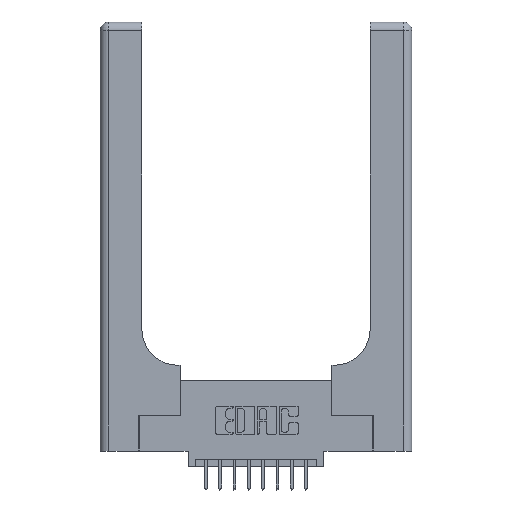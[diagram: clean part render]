
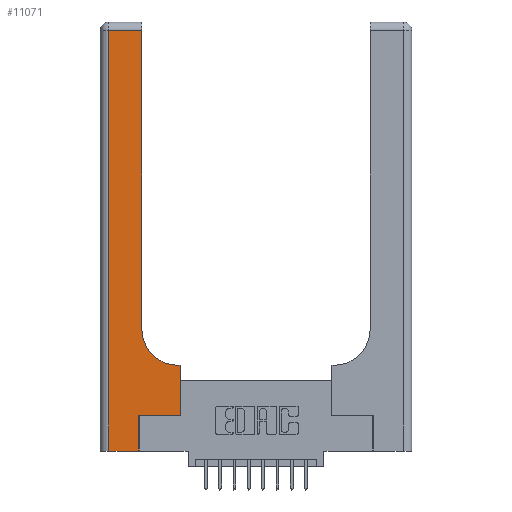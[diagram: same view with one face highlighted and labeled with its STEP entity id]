
A CAD part, top view. The second image highlights one B-rep face of the part: STEP entity #11071.
In plain terms, the highlighted planar face has unit normal (0, 0, 1).
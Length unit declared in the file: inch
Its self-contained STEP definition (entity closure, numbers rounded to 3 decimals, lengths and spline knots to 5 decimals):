
#88 = VERTEX_POINT ( 'NONE', #7089 ) ;
#295 = VECTOR ( 'NONE', #4574, 39.37008 ) ;
#316 = EDGE_CURVE ( 'NONE', #15069, #2921, #8820, .T. ) ;
#520 = PLANE ( 'NONE',  #4852 ) ;
#888 = LINE ( 'NONE', #1332, #7542 ) ;
#951 = EDGE_CURVE ( 'NONE', #16034, #15922, #11144, .T. ) ;
#986 = EDGE_CURVE ( 'NONE', #9569, #9562, #5456, .T. ) ;
#1092 = ORIENTED_EDGE ( 'NONE', *, *, #16101, .T. ) ;
#1332 = CARTESIAN_POINT ( 'NONE',  ( 0.2915, 3., 0.37 ) ) ;
#1518 = EDGE_CURVE ( 'NONE', #2921, #11020, #15280, .T. ) ;
#1629 = CARTESIAN_POINT ( 'NONE',  ( 0.06, 0., 0.37 ) ) ;
#1676 = DIRECTION ( 'NONE',  ( 0., 0., -1. ) ) ;
#2145 = DIRECTION ( 'NONE',  ( -1., 0., 0. ) ) ;
#2536 = VECTOR ( 'NONE', #2145, 39.37008 ) ;
#2921 = VERTEX_POINT ( 'NONE', #11684 ) ;
#4001 = CARTESIAN_POINT ( 'NONE',  ( 0.269, 0., 0.37 ) ) ;
#4333 = DIRECTION ( 'NONE',  ( -1., 0., 0. ) ) ;
#4574 = DIRECTION ( 'NONE',  ( 1., 0., 0. ) ) ;
#4661 = VECTOR ( 'NONE', #15684, 39.37008 ) ;
#4852 = AXIS2_PLACEMENT_3D ( 'NONE', #9300, #1676, #13098 ) ;
#4857 = VECTOR ( 'NONE', #5450, 39.37008 ) ;
#4906 = ORIENTED_EDGE ( 'NONE', *, *, #316, .T. ) ;
#5363 = DIRECTION ( 'NONE',  ( 1., 0., 0. ) ) ;
#5450 = DIRECTION ( 'NONE',  ( 0., -1., 0. ) ) ;
#5456 = LINE ( 'NONE', #9406, #4661 ) ;
#5468 = ORIENTED_EDGE ( 'NONE', *, *, #986, .T. ) ;
#5561 = VERTEX_POINT ( 'NONE', #4001 ) ;
#6009 = VECTOR ( 'NONE', #11252, 39.37008 ) ;
#6308 = DIRECTION ( 'NONE',  ( 0., 1., 0. ) ) ;
#6464 = CARTESIAN_POINT ( 'NONE',  ( 0.5585, 0.25, 0.37 ) ) ;
#6679 = CARTESIAN_POINT ( 'NONE',  ( 0., 2.94, 0.37 ) ) ;
#7070 = CARTESIAN_POINT ( 'NONE',  ( 0.2915, 0.6, 0.37 ) ) ;
#7089 = CARTESIAN_POINT ( 'NONE',  ( 0.2915, 2.94, 0.37 ) ) ;
#7542 = VECTOR ( 'NONE', #6308, 39.37008 ) ;
#7837 = CARTESIAN_POINT ( 'NONE',  ( 0.5415, 0.85, 0.37 ) ) ;
#7860 = LINE ( 'NONE', #6679, #16120 ) ;
#7873 = CARTESIAN_POINT ( 'NONE',  ( 0.06, 3., 0.37 ) ) ;
#7876 = VECTOR ( 'NONE', #11404, 39.37008 ) ;
#8270 = LINE ( 'NONE', #6464, #7876 ) ;
#8290 = EDGE_LOOP ( 'NONE', ( #9722, #14265, #12399, #10704, #1092, #5468, #15991, #4906, #9548 ) ) ;
#8411 = CARTESIAN_POINT ( 'NONE',  ( 0.269, 0., 0.37 ) ) ;
#8820 = LINE ( 'NONE', #7070, #2536 ) ;
#9149 = CARTESIAN_POINT ( 'NONE',  ( 0.269, 0.25, 0.37 ) ) ;
#9300 = CARTESIAN_POINT ( 'NONE',  ( 0., 3., 0.37 ) ) ;
#9326 = LINE ( 'NONE', #10823, #295 ) ;
#9406 = CARTESIAN_POINT ( 'NONE',  ( 0.269, 0.25, 0.37 ) ) ;
#9500 = CARTESIAN_POINT ( 'NONE',  ( 0.5585, 0.6, 0.37 ) ) ;
#9548 = ORIENTED_EDGE ( 'NONE', *, *, #1518, .T. ) ;
#9562 = VERTEX_POINT ( 'NONE', #10160 ) ;
#9569 = VERTEX_POINT ( 'NONE', #9149 ) ;
#9588 = EDGE_CURVE ( 'NONE', #15922, #5561, #9326, .T. ) ;
#9722 = ORIENTED_EDGE ( 'NONE', *, *, #16256, .T. ) ;
#10160 = CARTESIAN_POINT ( 'NONE',  ( 0.5585, 0.25, 0.37 ) ) ;
#10704 = ORIENTED_EDGE ( 'NONE', *, *, #9588, .T. ) ;
#10823 = CARTESIAN_POINT ( 'NONE',  ( 0., 0., 0.37 ) ) ;
#11020 = VERTEX_POINT ( 'NONE', #14228 ) ;
#11071 = ADVANCED_FACE ( 'NONE', ( #13222 ), #520, .F. ) ;
#11144 = LINE ( 'NONE', #7873, #4857 ) ;
#11252 = DIRECTION ( 'NONE',  ( 0., 1., 0. ) ) ;
#11404 = DIRECTION ( 'NONE',  ( 0., 1., 0. ) ) ;
#11684 = CARTESIAN_POINT ( 'NONE',  ( 0.5415, 0.6, 0.37 ) ) ;
#12010 = EDGE_CURVE ( 'NONE', #9562, #15069, #8270, .T. ) ;
#12242 = EDGE_CURVE ( 'NONE', #88, #16034, #7860, .T. ) ;
#12399 = ORIENTED_EDGE ( 'NONE', *, *, #951, .T. ) ;
#12736 = DIRECTION ( 'NONE',  ( 0., 0., -1. ) ) ;
#12802 = AXIS2_PLACEMENT_3D ( 'NONE', #7837, #12736, #5363 ) ;
#13098 = DIRECTION ( 'NONE',  ( -1., 0., 0. ) ) ;
#13222 = FACE_OUTER_BOUND ( 'NONE', #8290, .T. ) ;
#13919 = LINE ( 'NONE', #8411, #6009 ) ;
#14228 = CARTESIAN_POINT ( 'NONE',  ( 0.2915, 0.85, 0.37 ) ) ;
#14265 = ORIENTED_EDGE ( 'NONE', *, *, #12242, .T. ) ;
#15069 = VERTEX_POINT ( 'NONE', #9500 ) ;
#15280 = CIRCLE ( 'NONE', #12802, 0.25 ) ;
#15684 = DIRECTION ( 'NONE',  ( 1., 0., 0. ) ) ;
#15901 = CARTESIAN_POINT ( 'NONE',  ( 0.06, 2.94, 0.37 ) ) ;
#15922 = VERTEX_POINT ( 'NONE', #1629 ) ;
#15991 = ORIENTED_EDGE ( 'NONE', *, *, #12010, .T. ) ;
#16034 = VERTEX_POINT ( 'NONE', #15901 ) ;
#16101 = EDGE_CURVE ( 'NONE', #5561, #9569, #13919, .T. ) ;
#16120 = VECTOR ( 'NONE', #4333, 39.37008 ) ;
#16256 = EDGE_CURVE ( 'NONE', #11020, #88, #888, .T. ) ;
